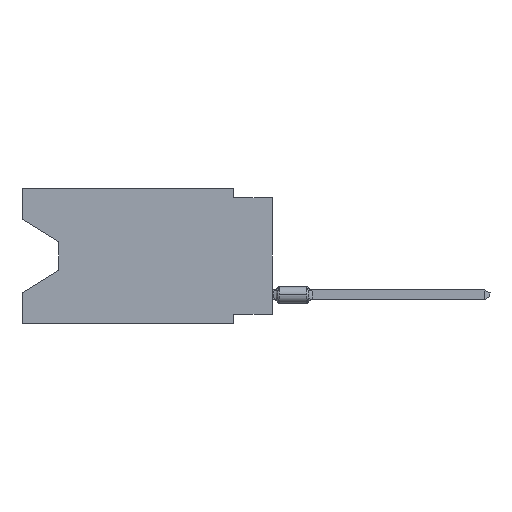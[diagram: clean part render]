
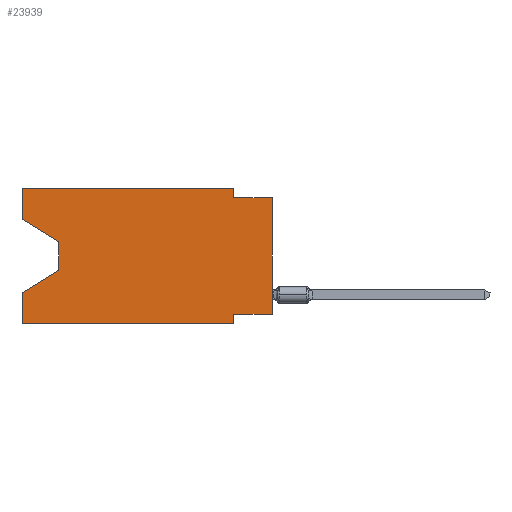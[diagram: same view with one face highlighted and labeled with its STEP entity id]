
A CAD part, left-side view. The second image highlights one B-rep face of the part: STEP entity #23939.
In plain terms, the highlighted planar face has unit normal (-1, 0, 0).
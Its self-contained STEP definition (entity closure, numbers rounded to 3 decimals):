
#867 = LINE ( 'NONE', #31020, #13947 ) ;
#1207 = VERTEX_POINT ( 'NONE', #16378 ) ;
#1308 = DIRECTION ( 'NONE',  ( 0., -0.855, -0.519 ) ) ;
#1779 = CARTESIAN_POINT ( 'NONE',  ( 0., 0., -0.635 ) ) ;
#1843 = ORIENTED_EDGE ( 'NONE', *, *, #39956, .T. ) ;
#2480 = CARTESIAN_POINT ( 'NONE',  ( 0., 2.54, 0. ) ) ;
#3780 = VECTOR ( 'NONE', #35982, 1000. ) ;
#4440 = FACE_OUTER_BOUND ( 'NONE', #19071, .T. ) ;
#5544 = EDGE_CURVE ( 'NONE', #1207, #14748, #867, .T. ) ;
#5558 = ORIENTED_EDGE ( 'NONE', *, *, #8718, .F. ) ;
#5807 = CARTESIAN_POINT ( 'NONE',  ( 0., 2.54, -8.89 ) ) ;
#8251 = VERTEX_POINT ( 'NONE', #38732 ) ;
#8698 = LINE ( 'NONE', #25895, #28931 ) ;
#8709 = CARTESIAN_POINT ( 'NONE',  ( 0., 0., 0. ) ) ;
#8718 = EDGE_CURVE ( 'NONE', #27195, #53570, #32006, .T. ) ;
#8879 = CARTESIAN_POINT ( 'NONE',  ( 0., 2.54, -0.635 ) ) ;
#9798 = CARTESIAN_POINT ( 'NONE',  ( 0., 16.383, 0. ) ) ;
#10200 = VECTOR ( 'NONE', #45862, 1000. ) ;
#12748 = CARTESIAN_POINT ( 'NONE',  ( 0., 2.54, -8.89 ) ) ;
#13947 = VECTOR ( 'NONE', #43726, 1000. ) ;
#14748 = VERTEX_POINT ( 'NONE', #41141 ) ;
#16378 = CARTESIAN_POINT ( 'NONE',  ( 0., 0., -8.255 ) ) ;
#17896 = DIRECTION ( 'NONE',  ( 0., -1., 0. ) ) ;
#18428 = ORIENTED_EDGE ( 'NONE', *, *, #5544, .F. ) ;
#18640 = EDGE_CURVE ( 'NONE', #34860, #32294, #50628, .T. ) ;
#18835 = LINE ( 'NONE', #9798, #53565 ) ;
#19009 = VECTOR ( 'NONE', #54885, 1000. ) ;
#19071 = EDGE_LOOP ( 'NONE', ( #29694, #50452, #45707, #54905, #1843, #47183, #18428, #32095, #5558, #27497, #42718, #28111 ) ) ;
#21493 = AXIS2_PLACEMENT_3D ( 'NONE', #38826, #51791, #21899 ) ;
#21845 = CARTESIAN_POINT ( 'NONE',  ( 0., 16.383, -8.89 ) ) ;
#21899 = DIRECTION ( 'NONE',  ( 0., 0., -1. ) ) ;
#22450 = CARTESIAN_POINT ( 'NONE',  ( 0., 16.383, 0. ) ) ;
#22796 = CARTESIAN_POINT ( 'NONE',  ( 0., 16.383, -6.852 ) ) ;
#22987 = CARTESIAN_POINT ( 'NONE',  ( 0., 16.383, 0. ) ) ;
#23242 = EDGE_CURVE ( 'NONE', #33654, #25796, #44197, .T. ) ;
#23274 = DIRECTION ( 'NONE',  ( 0., -1., 0. ) ) ;
#23699 = VERTEX_POINT ( 'NONE', #53132 ) ;
#23939 = ADVANCED_FACE ( 'NONE', ( #4440 ), #39093, .F. ) ;
#25772 = VECTOR ( 'NONE', #23274, 1000. ) ;
#25796 = VERTEX_POINT ( 'NONE', #22796 ) ;
#25868 = VECTOR ( 'NONE', #35748, 1000. ) ;
#25895 = CARTESIAN_POINT ( 'NONE',  ( 0., 13.97, -3.505 ) ) ;
#25904 = DIRECTION ( 'NONE',  ( 0., 0., 1. ) ) ;
#25938 = VECTOR ( 'NONE', #17896, 1000. ) ;
#27195 = VERTEX_POINT ( 'NONE', #8879 ) ;
#27497 = ORIENTED_EDGE ( 'NONE', *, *, #48087, .F. ) ;
#28111 = ORIENTED_EDGE ( 'NONE', *, *, #41187, .F. ) ;
#28657 = CARTESIAN_POINT ( 'NONE',  ( 0., 16.383, 0. ) ) ;
#28931 = VECTOR ( 'NONE', #34927, 1000. ) ;
#29247 = VECTOR ( 'NONE', #1308, 1000. ) ;
#29694 = ORIENTED_EDGE ( 'NONE', *, *, #54244, .T. ) ;
#30237 = LINE ( 'NONE', #12748, #32923 ) ;
#31020 = CARTESIAN_POINT ( 'NONE',  ( 0., 0., -8.255 ) ) ;
#32006 = LINE ( 'NONE', #49478, #25772 ) ;
#32095 = ORIENTED_EDGE ( 'NONE', *, *, #47829, .T. ) ;
#32294 = VERTEX_POINT ( 'NONE', #36093 ) ;
#32923 = VECTOR ( 'NONE', #47709, 1000. ) ;
#33654 = VERTEX_POINT ( 'NONE', #45784 ) ;
#34334 = VERTEX_POINT ( 'NONE', #55545 ) ;
#34860 = VERTEX_POINT ( 'NONE', #22987 ) ;
#34873 = LINE ( 'NONE', #22450, #3780 ) ;
#34927 = DIRECTION ( 'NONE',  ( 0., 0., -1. ) ) ;
#35452 = CARTESIAN_POINT ( 'NONE',  ( 0., 13.97, -5.385 ) ) ;
#35748 = DIRECTION ( 'NONE',  ( 0., 0.855, -0.519 ) ) ;
#35982 = DIRECTION ( 'NONE',  ( 0., 0., 1. ) ) ;
#36093 = CARTESIAN_POINT ( 'NONE',  ( 0., 2.54, 0. ) ) ;
#36284 = DIRECTION ( 'NONE',  ( 0., 0., 1. ) ) ;
#38732 = CARTESIAN_POINT ( 'NONE',  ( 0., 16.383, -2.038 ) ) ;
#38826 = CARTESIAN_POINT ( 'NONE',  ( 0., 16.383, 0. ) ) ;
#39040 = LINE ( 'NONE', #21845, #25938 ) ;
#39093 = PLANE ( 'NONE',  #21493 ) ;
#39921 = CARTESIAN_POINT ( 'NONE',  ( 0., 16.383, -2.038 ) ) ;
#39956 = EDGE_CURVE ( 'NONE', #23699, #50622, #39040, .T. ) ;
#41106 = LINE ( 'NONE', #2480, #19009 ) ;
#41141 = CARTESIAN_POINT ( 'NONE',  ( 0., 2.54, -8.255 ) ) ;
#41187 = EDGE_CURVE ( 'NONE', #8251, #34860, #18835, .T. ) ;
#42098 = EDGE_CURVE ( 'NONE', #14748, #50622, #30237, .T. ) ;
#42718 = ORIENTED_EDGE ( 'NONE', *, *, #18640, .F. ) ;
#43726 = DIRECTION ( 'NONE',  ( 0., 1., 0. ) ) ;
#43961 = LINE ( 'NONE', #8709, #52277 ) ;
#44197 = LINE ( 'NONE', #35452, #25868 ) ;
#44445 = LINE ( 'NONE', #39921, #29247 ) ;
#45707 = ORIENTED_EDGE ( 'NONE', *, *, #23242, .T. ) ;
#45784 = CARTESIAN_POINT ( 'NONE',  ( 0., 13.97, -5.385 ) ) ;
#45862 = DIRECTION ( 'NONE',  ( 0., -1., 0. ) ) ;
#46624 = EDGE_CURVE ( 'NONE', #34334, #33654, #8698, .T. ) ;
#47183 = ORIENTED_EDGE ( 'NONE', *, *, #42098, .F. ) ;
#47709 = DIRECTION ( 'NONE',  ( 0., 0., -1. ) ) ;
#47829 = EDGE_CURVE ( 'NONE', #1207, #53570, #43961, .T. ) ;
#48087 = EDGE_CURVE ( 'NONE', #32294, #27195, #41106, .T. ) ;
#49415 = EDGE_CURVE ( 'NONE', #23699, #25796, #34873, .T. ) ;
#49478 = CARTESIAN_POINT ( 'NONE',  ( 0., 0., -0.635 ) ) ;
#50452 = ORIENTED_EDGE ( 'NONE', *, *, #46624, .T. ) ;
#50622 = VERTEX_POINT ( 'NONE', #5807 ) ;
#50628 = LINE ( 'NONE', #28657, #10200 ) ;
#51791 = DIRECTION ( 'NONE',  ( 1., 0., 0. ) ) ;
#52277 = VECTOR ( 'NONE', #25904, 1000. ) ;
#53132 = CARTESIAN_POINT ( 'NONE',  ( 0., 16.383, -8.89 ) ) ;
#53565 = VECTOR ( 'NONE', #36284, 1000. ) ;
#53570 = VERTEX_POINT ( 'NONE', #1779 ) ;
#54244 = EDGE_CURVE ( 'NONE', #8251, #34334, #44445, .T. ) ;
#54885 = DIRECTION ( 'NONE',  ( 0., 0., -1. ) ) ;
#54905 = ORIENTED_EDGE ( 'NONE', *, *, #49415, .F. ) ;
#55545 = CARTESIAN_POINT ( 'NONE',  ( 0., 13.97, -3.505 ) ) ;
